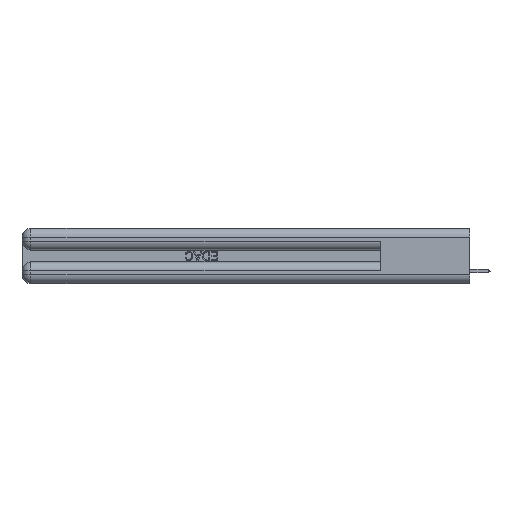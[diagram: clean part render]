
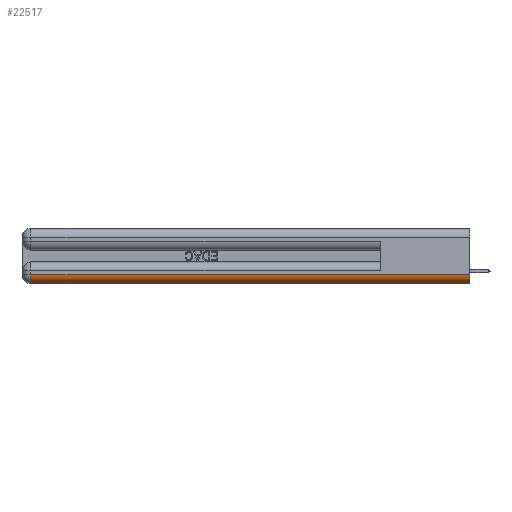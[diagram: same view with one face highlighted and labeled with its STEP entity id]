
A CAD part, left-side view. The second image highlights one B-rep face of the part: STEP entity #22517.
In plain terms, the highlighted cylindrical face has radius 1.524 mm (diameter 3.048 mm), a partial arc.
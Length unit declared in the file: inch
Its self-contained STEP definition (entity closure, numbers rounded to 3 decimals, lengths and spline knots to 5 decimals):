
#524 = VERTEX_POINT ( 'NONE', #17390 ) ;
#608 = EDGE_CURVE ( 'NONE', #30319, #18505, #10871, .T. ) ;
#1172 = ORIENTED_EDGE ( 'NONE', *, *, #6657, .F. ) ;
#5199 = CIRCLE ( 'NONE', #34197, 0.06 ) ;
#5869 = VECTOR ( 'NONE', #28255, 39.37008 ) ;
#6369 = EDGE_CURVE ( 'NONE', #524, #30319, #24197, .T. ) ;
#6657 = EDGE_CURVE ( 'NONE', #18505, #21336, #7015, .T. ) ;
#7015 = LINE ( 'NONE', #20967, #5869 ) ;
#8071 = DIRECTION ( 'NONE',  ( 0., 0., 1. ) ) ;
#8741 = DIRECTION ( 'NONE',  ( 0., 0., 1. ) ) ;
#10370 = CYLINDRICAL_SURFACE ( 'NONE', #25204, 0.06 ) ;
#10871 = CIRCLE ( 'NONE', #25877, 0.06 ) ;
#13820 = CARTESIAN_POINT ( 'NONE',  ( 0., 2.94, 0.06 ) ) ;
#15522 = CARTESIAN_POINT ( 'NONE',  ( 0.06, 2.94, 0.06 ) ) ;
#16206 = ORIENTED_EDGE ( 'NONE', *, *, #33005, .F. ) ;
#17390 = CARTESIAN_POINT ( 'NONE',  ( 0.06, 0., 0. ) ) ;
#18505 = VERTEX_POINT ( 'NONE', #13820 ) ;
#20967 = CARTESIAN_POINT ( 'NONE',  ( 0., 0., 0.06 ) ) ;
#21336 = VERTEX_POINT ( 'NONE', #44904 ) ;
#22377 = CARTESIAN_POINT ( 'NONE',  ( 0.06, 0., 0.06 ) ) ;
#22460 = ORIENTED_EDGE ( 'NONE', *, *, #6369, .F. ) ;
#22517 = ADVANCED_FACE ( 'NONE', ( #40654 ), #10370, .T. ) ;
#23249 = DIRECTION ( 'NONE',  ( 0., 1., 0. ) ) ;
#23530 = DIRECTION ( 'NONE',  ( 0., -1., 0. ) ) ;
#24197 = LINE ( 'NONE', #29660, #33098 ) ;
#25104 = ORIENTED_EDGE ( 'NONE', *, *, #608, .F. ) ;
#25204 = AXIS2_PLACEMENT_3D ( 'NONE', #22377, #48911, #26129 ) ;
#25877 = AXIS2_PLACEMENT_3D ( 'NONE', #15522, #38402, #8071 ) ;
#26129 = DIRECTION ( 'NONE',  ( 0., 0., 1. ) ) ;
#28255 = DIRECTION ( 'NONE',  ( 0., -1., 0. ) ) ;
#29660 = CARTESIAN_POINT ( 'NONE',  ( 0.06, 3., 0. ) ) ;
#30319 = VERTEX_POINT ( 'NONE', #45142 ) ;
#33005 = EDGE_CURVE ( 'NONE', #21336, #524, #5199, .T. ) ;
#33098 = VECTOR ( 'NONE', #23249, 39.37008 ) ;
#34197 = AXIS2_PLACEMENT_3D ( 'NONE', #42623, #23530, #8741 ) ;
#38402 = DIRECTION ( 'NONE',  ( 0., 1., 0. ) ) ;
#40654 = FACE_OUTER_BOUND ( 'NONE', #48622, .T. ) ;
#42623 = CARTESIAN_POINT ( 'NONE',  ( 0.06, 0., 0.06 ) ) ;
#44904 = CARTESIAN_POINT ( 'NONE',  ( 0., 0., 0.06 ) ) ;
#45142 = CARTESIAN_POINT ( 'NONE',  ( 0.06, 2.94, 0. ) ) ;
#48622 = EDGE_LOOP ( 'NONE', ( #16206, #1172, #25104, #22460 ) ) ;
#48911 = DIRECTION ( 'NONE',  ( 0., 1., 0. ) ) ;
